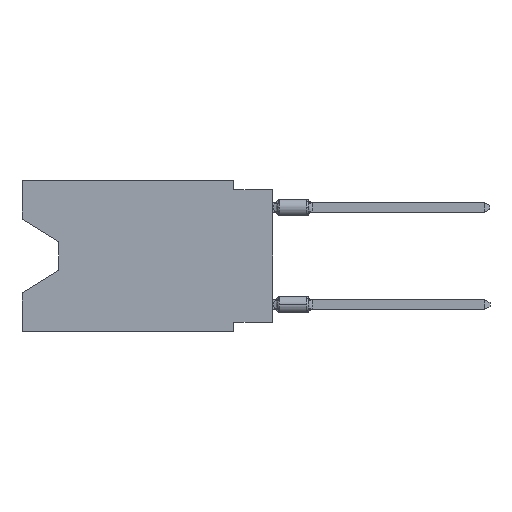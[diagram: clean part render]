
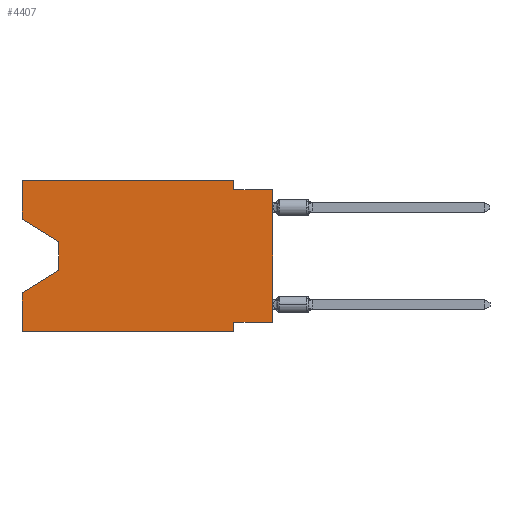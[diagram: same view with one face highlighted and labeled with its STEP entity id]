
A CAD part, left-side view. The second image highlights one B-rep face of the part: STEP entity #4407.
In plain terms, the highlighted planar face has unit normal (-1, 0, 0).
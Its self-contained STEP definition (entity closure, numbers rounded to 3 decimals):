
#10 = CARTESIAN_POINT ( 'NONE',  ( 0., 2.54, -0.635 ) ) ;
#536 = PLANE ( 'NONE',  #23706 ) ;
#555 = LINE ( 'NONE', #4242, #18532 ) ;
#692 = DIRECTION ( 'NONE',  ( 0., 0., 1. ) ) ;
#1099 = LINE ( 'NONE', #4409, #21682 ) ;
#1400 = VECTOR ( 'NONE', #2621, 1000. ) ;
#1922 = DIRECTION ( 'NONE',  ( 0., 0., 1. ) ) ;
#1959 = EDGE_CURVE ( 'NONE', #10452, #16867, #21428, .T. ) ;
#2013 = EDGE_CURVE ( 'NONE', #16402, #19453, #1099, .T. ) ;
#2127 = ORIENTED_EDGE ( 'NONE', *, *, #22207, .F. ) ;
#2451 = DIRECTION ( 'NONE',  ( 0., 0., -1. ) ) ;
#2593 = DIRECTION ( 'NONE',  ( 0., 0., 1. ) ) ;
#2621 = DIRECTION ( 'NONE',  ( 0., -1., 0. ) ) ;
#2964 = VERTEX_POINT ( 'NONE', #21604 ) ;
#3204 = ORIENTED_EDGE ( 'NONE', *, *, #15356, .T. ) ;
#3562 = ORIENTED_EDGE ( 'NONE', *, *, #1959, .F. ) ;
#4064 = CARTESIAN_POINT ( 'NONE',  ( 0., 0., -0.635 ) ) ;
#4093 = ORIENTED_EDGE ( 'NONE', *, *, #19982, .F. ) ;
#4164 = VECTOR ( 'NONE', #5299, 1000. ) ;
#4242 = CARTESIAN_POINT ( 'NONE',  ( 0., 16.383, 0. ) ) ;
#4407 = ADVANCED_FACE ( 'NONE', ( #22959 ), #536, .F. ) ;
#4409 = CARTESIAN_POINT ( 'NONE',  ( 0., 16.383, -2.546 ) ) ;
#4459 = VECTOR ( 'NONE', #1922, 1000. ) ;
#4493 = VECTOR ( 'NONE', #20611, 1000. ) ;
#5299 = DIRECTION ( 'NONE',  ( 0., 1., 0. ) ) ;
#5771 = ORIENTED_EDGE ( 'NONE', *, *, #16340, .F. ) ;
#6665 = ORIENTED_EDGE ( 'NONE', *, *, #12626, .T. ) ;
#7008 = CARTESIAN_POINT ( 'NONE',  ( 0., 0., -9.271 ) ) ;
#7078 = CARTESIAN_POINT ( 'NONE',  ( 0., 0., -0.635 ) ) ;
#7109 = ORIENTED_EDGE ( 'NONE', *, *, #21852, .F. ) ;
#7130 = CARTESIAN_POINT ( 'NONE',  ( 0., 16.383, 0. ) ) ;
#7429 = LINE ( 'NONE', #7078, #9846 ) ;
#7434 = VERTEX_POINT ( 'NONE', #7130 ) ;
#7844 = LINE ( 'NONE', #18762, #4493 ) ;
#8118 = LINE ( 'NONE', #17430, #1400 ) ;
#8122 = CARTESIAN_POINT ( 'NONE',  ( 0., 16.383, 0. ) ) ;
#8450 = CARTESIAN_POINT ( 'NONE',  ( 0., 16.383, -9.906 ) ) ;
#8805 = DIRECTION ( 'NONE',  ( 0., -1., 0. ) ) ;
#9846 = VECTOR ( 'NONE', #8805, 1000. ) ;
#9920 = LINE ( 'NONE', #22787, #20800 ) ;
#10452 = VERTEX_POINT ( 'NONE', #21457 ) ;
#11525 = ORIENTED_EDGE ( 'NONE', *, *, #21160, .T. ) ;
#11904 = DIRECTION ( 'NONE',  ( 0., 0., -1. ) ) ;
#11945 = DIRECTION ( 'NONE',  ( 1., 0., 0. ) ) ;
#12044 = CARTESIAN_POINT ( 'NONE',  ( 0., 0., 0. ) ) ;
#12232 = CARTESIAN_POINT ( 'NONE',  ( 0., 2.54, 0. ) ) ;
#12513 = VERTEX_POINT ( 'NONE', #10 ) ;
#12626 = EDGE_CURVE ( 'NONE', #19453, #22166, #17390, .T. ) ;
#13084 = CARTESIAN_POINT ( 'NONE',  ( 0., 16.383, 0. ) ) ;
#13492 = VECTOR ( 'NONE', #23141, 1000. ) ;
#13608 = ORIENTED_EDGE ( 'NONE', *, *, #15542, .T. ) ;
#13894 = CARTESIAN_POINT ( 'NONE',  ( 0., 16.383, -7.36 ) ) ;
#14270 = VECTOR ( 'NONE', #15911, 1000. ) ;
#14712 = CARTESIAN_POINT ( 'NONE',  ( 0., 16.383, -2.546 ) ) ;
#14722 = VECTOR ( 'NONE', #2451, 1000. ) ;
#15005 = VERTEX_POINT ( 'NONE', #13894 ) ;
#15356 = EDGE_CURVE ( 'NONE', #22166, #15005, #7844, .T. ) ;
#15435 = CARTESIAN_POINT ( 'NONE',  ( 0., 13.97, -5.893 ) ) ;
#15542 = EDGE_CURVE ( 'NONE', #2964, #17737, #21327, .T. ) ;
#15911 = DIRECTION ( 'NONE',  ( 0., -1., 0. ) ) ;
#16021 = CARTESIAN_POINT ( 'NONE',  ( 0., 2.54, -9.906 ) ) ;
#16340 = EDGE_CURVE ( 'NONE', #2964, #10452, #18394, .T. ) ;
#16402 = VERTEX_POINT ( 'NONE', #14712 ) ;
#16867 = VERTEX_POINT ( 'NONE', #23632 ) ;
#17251 = ORIENTED_EDGE ( 'NONE', *, *, #19861, .F. ) ;
#17390 = LINE ( 'NONE', #18753, #14722 ) ;
#17430 = CARTESIAN_POINT ( 'NONE',  ( 0., 16.383, 0. ) ) ;
#17509 = DIRECTION ( 'NONE',  ( 0., -0.855, -0.519 ) ) ;
#17737 = VERTEX_POINT ( 'NONE', #4064 ) ;
#17746 = LINE ( 'NONE', #8450, #14270 ) ;
#18394 = LINE ( 'NONE', #7008, #4164 ) ;
#18505 = EDGE_LOOP ( 'NONE', ( #22432, #6665, #3204, #17251, #11525, #3562, #5771, #13608, #20195, #2127, #7109, #4093 ) ) ;
#18522 = CARTESIAN_POINT ( 'NONE',  ( 0., 13.97, -4.013 ) ) ;
#18532 = VECTOR ( 'NONE', #692, 1000. ) ;
#18753 = CARTESIAN_POINT ( 'NONE',  ( 0., 13.97, -4.013 ) ) ;
#18762 = CARTESIAN_POINT ( 'NONE',  ( 0., 13.97, -5.893 ) ) ;
#19413 = DIRECTION ( 'NONE',  ( 0., 0., -1. ) ) ;
#19453 = VERTEX_POINT ( 'NONE', #18522 ) ;
#19861 = EDGE_CURVE ( 'NONE', #21370, #15005, #22633, .T. ) ;
#19982 = EDGE_CURVE ( 'NONE', #16402, #7434, #555, .T. ) ;
#20195 = ORIENTED_EDGE ( 'NONE', *, *, #22454, .F. ) ;
#20611 = DIRECTION ( 'NONE',  ( 0., 0.855, -0.519 ) ) ;
#20798 = CARTESIAN_POINT ( 'NONE',  ( 0., 16.383, -9.906 ) ) ;
#20800 = VECTOR ( 'NONE', #11904, 1000. ) ;
#20944 = VECTOR ( 'NONE', #2593, 1000. ) ;
#21160 = EDGE_CURVE ( 'NONE', #21370, #16867, #17746, .T. ) ;
#21327 = LINE ( 'NONE', #12044, #20944 ) ;
#21370 = VERTEX_POINT ( 'NONE', #20798 ) ;
#21428 = LINE ( 'NONE', #16021, #13492 ) ;
#21457 = CARTESIAN_POINT ( 'NONE',  ( 0., 2.54, -9.271 ) ) ;
#21604 = CARTESIAN_POINT ( 'NONE',  ( 0., 0., -9.271 ) ) ;
#21682 = VECTOR ( 'NONE', #17509, 1000. ) ;
#21852 = EDGE_CURVE ( 'NONE', #7434, #22696, #8118, .T. ) ;
#22166 = VERTEX_POINT ( 'NONE', #15435 ) ;
#22207 = EDGE_CURVE ( 'NONE', #22696, #12513, #9920, .T. ) ;
#22432 = ORIENTED_EDGE ( 'NONE', *, *, #2013, .T. ) ;
#22454 = EDGE_CURVE ( 'NONE', #12513, #17737, #7429, .T. ) ;
#22633 = LINE ( 'NONE', #13084, #4459 ) ;
#22696 = VERTEX_POINT ( 'NONE', #12232 ) ;
#22787 = CARTESIAN_POINT ( 'NONE',  ( 0., 2.54, 0. ) ) ;
#22959 = FACE_OUTER_BOUND ( 'NONE', #18505, .T. ) ;
#23141 = DIRECTION ( 'NONE',  ( 0., 0., -1. ) ) ;
#23632 = CARTESIAN_POINT ( 'NONE',  ( 0., 2.54, -9.906 ) ) ;
#23706 = AXIS2_PLACEMENT_3D ( 'NONE', #8122, #11945, #19413 ) ;
